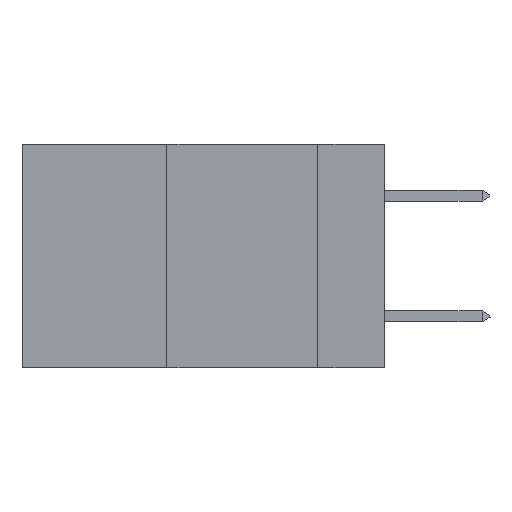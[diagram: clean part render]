
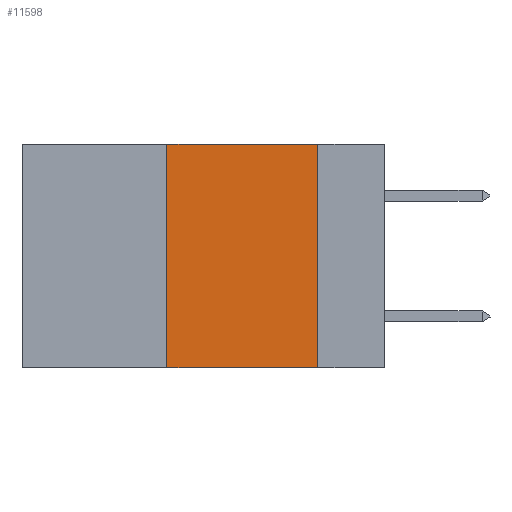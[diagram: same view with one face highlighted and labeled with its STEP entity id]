
A CAD part, left-side view. The second image highlights one B-rep face of the part: STEP entity #11598.
In plain terms, the highlighted planar face has unit normal (-1, 0, 0).
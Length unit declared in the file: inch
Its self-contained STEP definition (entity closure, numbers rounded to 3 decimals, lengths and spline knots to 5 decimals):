
#1592 = CARTESIAN_POINT ( 'NONE',  ( 0., 0.36, 0. ) ) ;
#2225 = EDGE_LOOP ( 'NONE', ( #38569, #7529, #26018, #34275 ) ) ;
#2236 = LINE ( 'NONE', #36510, #18190 ) ;
#3750 = AXIS2_PLACEMENT_3D ( 'NONE', #24199, #10803, #7293 ) ;
#4865 = FACE_OUTER_BOUND ( 'NONE', #2225, .T. ) ;
#7293 = DIRECTION ( 'NONE',  ( 0., 0., -1. ) ) ;
#7529 = ORIENTED_EDGE ( 'NONE', *, *, #38055, .F. ) ;
#7932 = VERTEX_POINT ( 'NONE', #32304 ) ;
#8123 = VECTOR ( 'NONE', #30868, 39.37008 ) ;
#9282 = DIRECTION ( 'NONE',  ( 0., -1., 0. ) ) ;
#9406 = VERTEX_POINT ( 'NONE', #42853 ) ;
#10038 = CARTESIAN_POINT ( 'NONE',  ( 0., 0.36, 0. ) ) ;
#10803 = DIRECTION ( 'NONE',  ( 1., 0., 0. ) ) ;
#11598 = ADVANCED_FACE ( 'NONE', ( #4865 ), #41555, .F. ) ;
#13730 = LINE ( 'NONE', #17669, #8123 ) ;
#14209 = EDGE_CURVE ( 'NONE', #7932, #24921, #13730, .T. ) ;
#15382 = CARTESIAN_POINT ( 'NONE',  ( 0., 0.11, -0.37 ) ) ;
#17669 = CARTESIAN_POINT ( 'NONE',  ( 0., 0.11, 0. ) ) ;
#18190 = VECTOR ( 'NONE', #9282, 39.37008 ) ;
#18989 = LINE ( 'NONE', #32384, #38410 ) ;
#22114 = EDGE_CURVE ( 'NONE', #9406, #25586, #27175, .T. ) ;
#24199 = CARTESIAN_POINT ( 'NONE',  ( 0., 0.6, 0. ) ) ;
#24921 = VERTEX_POINT ( 'NONE', #15382 ) ;
#25586 = VERTEX_POINT ( 'NONE', #1592 ) ;
#26018 = ORIENTED_EDGE ( 'NONE', *, *, #22114, .F. ) ;
#27175 = LINE ( 'NONE', #10038, #39489 ) ;
#30868 = DIRECTION ( 'NONE',  ( 0., 0., -1. ) ) ;
#30906 = EDGE_CURVE ( 'NONE', #9406, #24921, #2236, .T. ) ;
#32304 = CARTESIAN_POINT ( 'NONE',  ( 0., 0.11, 0. ) ) ;
#32384 = CARTESIAN_POINT ( 'NONE',  ( 0., 0.6, 0. ) ) ;
#34275 = ORIENTED_EDGE ( 'NONE', *, *, #30906, .T. ) ;
#36121 = DIRECTION ( 'NONE',  ( 0., -1., 0. ) ) ;
#36510 = CARTESIAN_POINT ( 'NONE',  ( 0., 0.6, -0.37 ) ) ;
#38055 = EDGE_CURVE ( 'NONE', #25586, #7932, #18989, .T. ) ;
#38410 = VECTOR ( 'NONE', #36121, 39.37008 ) ;
#38569 = ORIENTED_EDGE ( 'NONE', *, *, #14209, .F. ) ;
#39489 = VECTOR ( 'NONE', #40572, 39.37008 ) ;
#40572 = DIRECTION ( 'NONE',  ( 0., 0., 1. ) ) ;
#41555 = PLANE ( 'NONE',  #3750 ) ;
#42853 = CARTESIAN_POINT ( 'NONE',  ( 0., 0.36, -0.37 ) ) ;
